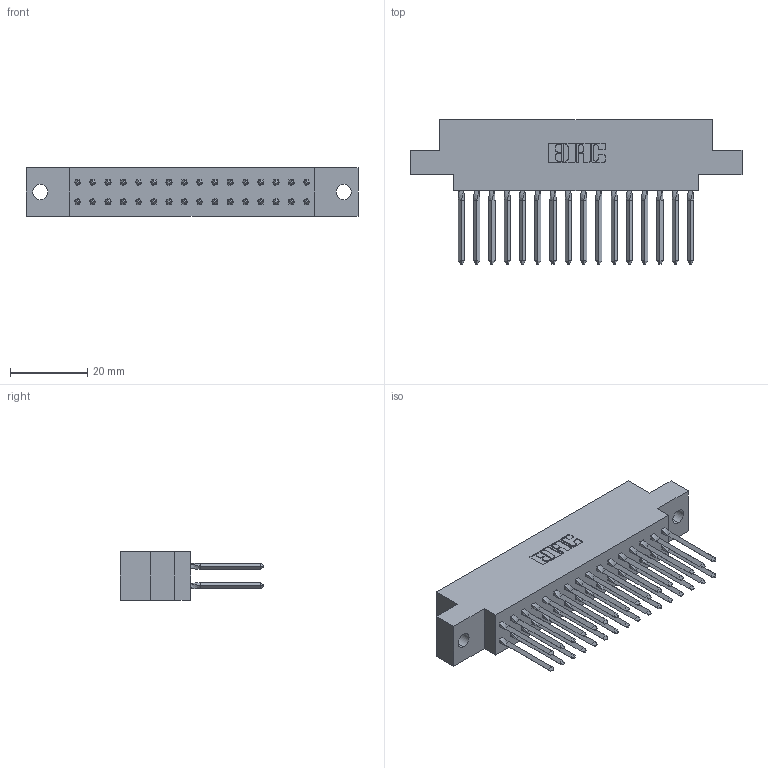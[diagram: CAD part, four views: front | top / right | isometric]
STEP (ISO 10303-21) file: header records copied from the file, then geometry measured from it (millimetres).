
FILE_DESCRIPTION (( 'STEP AP203' ), '1' );
FILE_NAME ('317-032-542-804.STEP', '2020-02-27T21:14:28', ( '' ), ( '' ), 'SwSTEP 2.0', 'SolidWorks 2016', '' );
FILE_SCHEMA (( 'CONFIG_CONTROL_DESIGN' ));
Length unit declared in the file: inch
Products named in the file (3): 317-032-542-804; 317 Part_.156 Dia - TH; 317-290-003_542
Assembly tree (33 placements, depth 2):
  317-032-542-804
    317 Part_.156 Dia - TH
    317-290-003_542  x32
Bounding box: 86.11 x 37.34 x 12.7 mm (x, y, z)
Volume: 13190 mm3; surface area: 17324.8 mm2
Topology: 33 solids, 33 shells, 1926 faces, 5395 edges, 3446 vertices
Faces by surface type: plane 1530, cylinder 268, bspline 128
Entity records: 25775 total; most frequent: CARTESIAN_POINT 4741, ORIENTED_EDGE 4404, DIRECTION 3750, EDGE_CURVE 2202, LINE 2032, VECTOR 2032, VERTEX_POINT 1462, AXIS2_PLACEMENT_3D 859
